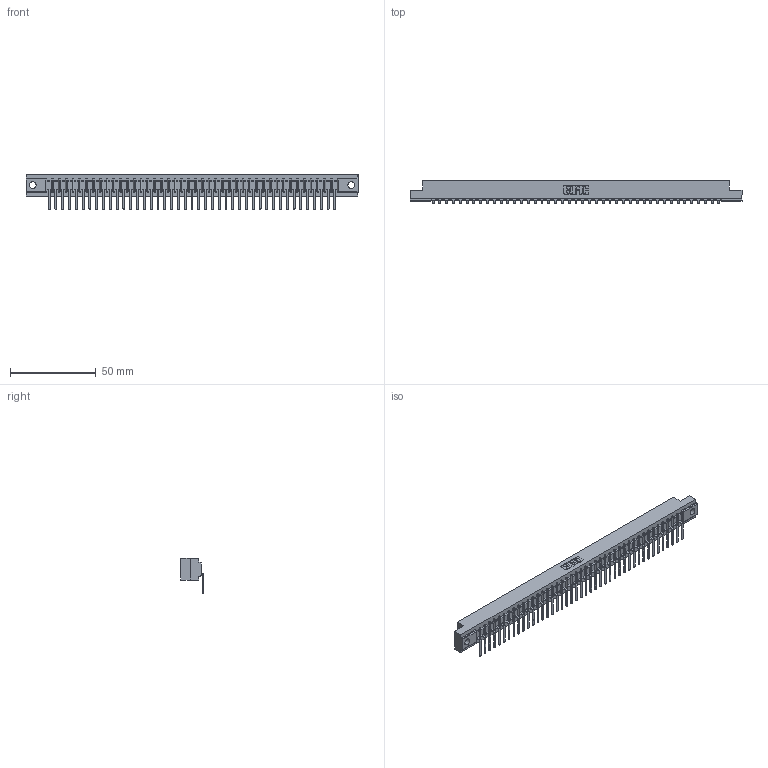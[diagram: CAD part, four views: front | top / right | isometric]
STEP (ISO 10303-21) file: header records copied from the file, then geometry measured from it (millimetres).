
FILE_DESCRIPTION (( 'STEP AP203' ), '1' );
FILE_NAME ('307-043-557-104.STEP', '2018-08-06T01:03:10', ( '' ), ( '' ), 'SwSTEP 2.0', 'SolidWorks 2016', '' );
FILE_SCHEMA (( 'CONFIG_CONTROL_DESIGN' ));
Length unit declared in the file: inch
Products named in the file (3): 307-043-557-104; 307 Part_.156 Dia Mounting Holes; 307-290-002_557
Assembly tree (44 placements, depth 2):
  307-043-557-104
    307 Part_.156 Dia Mounting Holes
    307-290-002_557  x43
Bounding box: 193.4 x 13.32 x 20.66 mm (x, y, z)
Volume: 20713.3 mm3; surface area: 26655.9 mm2
Topology: 44 solids, 44 shells, 3530 faces, 10851 edges, 7114 vertices
Faces by surface type: plane 2105, cylinder 1337, sphere 88
Entity records: 38012 total; most frequent: CARTESIAN_POINT 6418, ORIENTED_EDGE 6406, DIRECTION 6227, EDGE_CURVE 3203, LINE 2461, VECTOR 2461, VERTEX_POINT 2074, AXIS2_PLACEMENT_3D 1883
